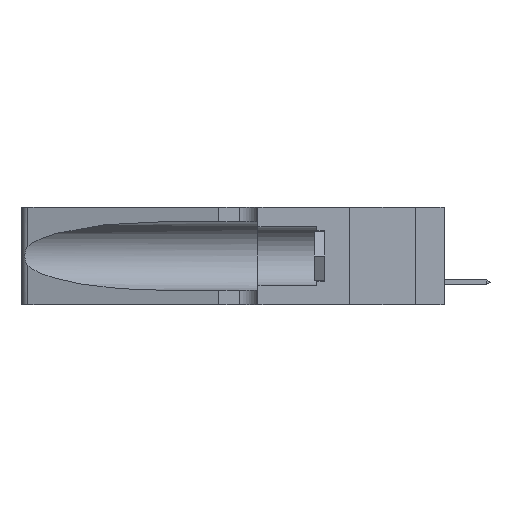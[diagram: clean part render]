
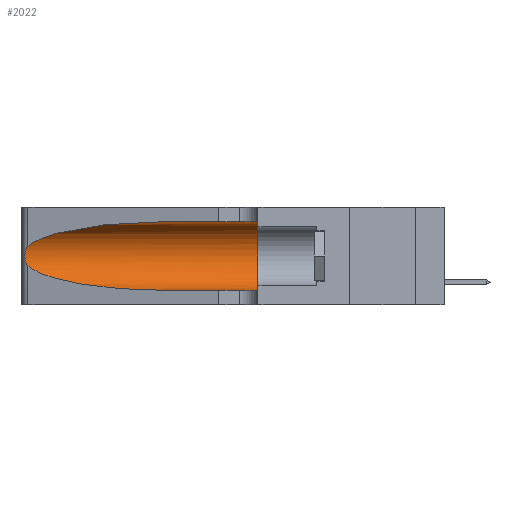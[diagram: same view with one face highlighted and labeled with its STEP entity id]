
A CAD part, left-side view. The second image highlights one B-rep face of the part: STEP entity #2022.
In plain terms, the highlighted cylindrical face has radius 3.308 mm (diameter 6.617 mm), a partial arc.
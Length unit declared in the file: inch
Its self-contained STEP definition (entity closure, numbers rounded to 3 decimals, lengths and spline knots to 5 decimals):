
#895 = CARTESIAN_POINT ( 'NONE',  ( 0.26075, 1.23896, 0.178 ) ) ;
#1084 = CARTESIAN_POINT ( 'NONE',  ( 0.25789, 1.23486, 0.15765 ) ) ;
#1681 = CARTESIAN_POINT ( 'NONE',  ( 0.1305, 1.61858, 0.05475 ) ) ;
#2022 = ADVANCED_FACE ( 'NONE', ( #19001 ), #25500, .F. ) ;
#2192 = CARTESIAN_POINT ( 'NONE',  ( 0.1305, 0.35, 0.31525 ) ) ;
#3175 = CARTESIAN_POINT ( 'NONE',  ( 0.26017, 1.23833, 0.17102 ) ) ;
#3260 = CARTESIAN_POINT ( 'NONE',  ( 0.25487, 1.22718, 0.22369 ) ) ;
#3680 = CARTESIAN_POINT ( 'NONE',  ( 0.18966, 0.96281, 0.05475 ) ) ;
#4371 = EDGE_CURVE ( 'NONE', #13887, #6956, #28282, .T. ) ;
#4872 = DIRECTION ( 'NONE',  ( 0., 1., 0. ) ) ;
#5589 = EDGE_LOOP ( 'NONE', ( #8509, #25087, #11825, #19146, #22375, #6276 ) ) ;
#6276 = ORIENTED_EDGE ( 'NONE', *, *, #19593, .F. ) ;
#6299 = CARTESIAN_POINT ( 'NONE',  ( 0.1305, 0.72297, 0.31525 ) ) ;
#6349 = AXIS2_PLACEMENT_3D ( 'NONE', #23800, #17029, #8109 ) ;
#6956 = VERTEX_POINT ( 'NONE', #27412 ) ;
#7558 = CARTESIAN_POINT ( 'NONE',  ( 0.25555, 1.22993, 0.14849 ) ) ;
#7733 = CARTESIAN_POINT ( 'NONE',  ( 0.1305, 0.72297, 0.31525 ) ) ;
#8109 = DIRECTION ( 'NONE',  ( 0., 0., -1. ) ) ;
#8509 = ORIENTED_EDGE ( 'NONE', *, *, #13877, .T. ) ;
#8916 =( BOUNDED_CURVE ( )  B_SPLINE_CURVE ( 3, ( #16526, #25225, #3680, #21270 ),
 .UNSPECIFIED., .F., .F. ) 
 B_SPLINE_CURVE_WITH_KNOTS ( ( 4, 4 ),
 ( 3.44316, 4.71239 ),
 .UNSPECIFIED. ) 
 CURVE ( )  GEOMETRIC_REPRESENTATION_ITEM ( )  RATIONAL_B_SPLINE_CURVE ( ( 1., 0.87, 0.87, 1. ) ) 
 REPRESENTATION_ITEM ( '' )  );
#9267 = B_SPLINE_CURVE_WITH_KNOTS ( 'NONE', 3,
 ( #3260, #11821, #18405, #27222, #18689, #11726, #27312, #895, #3175, #18597, #1084, #20752, #7558, #9755 ),
 .UNSPECIFIED., .F., .F.,
 ( 4, 2, 2, 2, 2, 2, 4 ),
 ( 0., 0.00027, 0.00053, 0.00107, 0.0016, 0.00187, 0.00214 ),
 .UNSPECIFIED. ) ;
#9755 = CARTESIAN_POINT ( 'NONE',  ( 0.25487, 1.22718, 0.14631 ) ) ;
#10133 = CARTESIAN_POINT ( 'NONE',  ( 0.1305, 0.72297, 0.05475 ) ) ;
#10475 = DIRECTION ( 'NONE',  ( 0., -1., 0. ) ) ;
#10984 = AXIS2_PLACEMENT_3D ( 'NONE', #11786, #4872, #26999 ) ;
#11726 = CARTESIAN_POINT ( 'NONE',  ( 0.26018, 1.23835, 0.19895 ) ) ;
#11786 = CARTESIAN_POINT ( 'NONE',  ( 0.1305, 0.35, 0.185 ) ) ;
#11821 = CARTESIAN_POINT ( 'NONE',  ( 0.25555, 1.22994, 0.2215 ) ) ;
#11825 = ORIENTED_EDGE ( 'NONE', *, *, #28073, .T. ) ;
#12923 = CARTESIAN_POINT ( 'NONE',  ( 0.2373, 1.15595, 0.28018 ) ) ;
#13802 = VERTEX_POINT ( 'NONE', #10133 ) ;
#13877 = EDGE_CURVE ( 'NONE', #22145, #16913, #20389, .T. ) ;
#13887 = VERTEX_POINT ( 'NONE', #2192 ) ;
#14227 = EDGE_CURVE ( 'NONE', #13802, #6956, #16659, .T. ) ;
#14651 = CARTESIAN_POINT ( 'NONE',  ( 0.1305, 1.61858, 0.31525 ) ) ;
#14879 = CARTESIAN_POINT ( 'NONE',  ( 0.25487, 1.22718, 0.14631 ) ) ;
#15415 = VECTOR ( 'NONE', #19107, 39.37008 ) ;
#15669 = CARTESIAN_POINT ( 'NONE',  ( 0.25487, 1.22718, 0.22369 ) ) ;
#15785 = LINE ( 'NONE', #14651, #15415 ) ;
#16526 = CARTESIAN_POINT ( 'NONE',  ( 0.25487, 1.22718, 0.14631 ) ) ;
#16659 = LINE ( 'NONE', #1681, #26252 ) ;
#16913 = VERTEX_POINT ( 'NONE', #15669 ) ;
#17029 = DIRECTION ( 'NONE',  ( 0., -1., 0. ) ) ;
#18405 = CARTESIAN_POINT ( 'NONE',  ( 0.25639, 1.23184, 0.21858 ) ) ;
#18597 = CARTESIAN_POINT ( 'NONE',  ( 0.25856, 1.23593, 0.16098 ) ) ;
#18689 = CARTESIAN_POINT ( 'NONE',  ( 0.25854, 1.2359, 0.20912 ) ) ;
#19001 = FACE_OUTER_BOUND ( 'NONE', #5589, .T. ) ;
#19107 = DIRECTION ( 'NONE',  ( 0., -1., 0. ) ) ;
#19146 = ORIENTED_EDGE ( 'NONE', *, *, #14227, .T. ) ;
#19593 = EDGE_CURVE ( 'NONE', #22145, #13887, #15785, .T. ) ;
#19798 = EDGE_CURVE ( 'NONE', #16913, #27651, #9267, .T. ) ;
#20389 =( BOUNDED_CURVE ( )  B_SPLINE_CURVE ( 3, ( #6299, #23693, #12923, #24080 ),
 .UNSPECIFIED., .F., .T. ) 
 B_SPLINE_CURVE_WITH_KNOTS ( ( 4, 4 ),
 ( 1.5708, 2.84003 ),
 .UNSPECIFIED. ) 
 CURVE ( )  GEOMETRIC_REPRESENTATION_ITEM ( )  RATIONAL_B_SPLINE_CURVE ( ( 1., 0.87, 0.87, 1. ) ) 
 REPRESENTATION_ITEM ( '' )  );
#20752 = CARTESIAN_POINT ( 'NONE',  ( 0.25639, 1.23186, 0.15144 ) ) ;
#21270 = CARTESIAN_POINT ( 'NONE',  ( 0.1305, 0.72297, 0.05475 ) ) ;
#22145 = VERTEX_POINT ( 'NONE', #7733 ) ;
#22375 = ORIENTED_EDGE ( 'NONE', *, *, #4371, .F. ) ;
#23693 = CARTESIAN_POINT ( 'NONE',  ( 0.18966, 0.96281, 0.31525 ) ) ;
#23800 = CARTESIAN_POINT ( 'NONE',  ( 0.1305, 1.61858, 0.185 ) ) ;
#24080 = CARTESIAN_POINT ( 'NONE',  ( 0.25487, 1.22718, 0.22369 ) ) ;
#25087 = ORIENTED_EDGE ( 'NONE', *, *, #19798, .T. ) ;
#25225 = CARTESIAN_POINT ( 'NONE',  ( 0.2373, 1.15595, 0.08982 ) ) ;
#25500 = CYLINDRICAL_SURFACE ( 'NONE', #6349, 0.13025 ) ;
#26252 = VECTOR ( 'NONE', #10475, 39.37008 ) ;
#26999 = DIRECTION ( 'NONE',  ( 0., 0., 1. ) ) ;
#27222 = CARTESIAN_POINT ( 'NONE',  ( 0.25787, 1.23484, 0.2124 ) ) ;
#27312 = CARTESIAN_POINT ( 'NONE',  ( 0.26075, 1.23896, 0.19203 ) ) ;
#27412 = CARTESIAN_POINT ( 'NONE',  ( 0.1305, 0.35, 0.05475 ) ) ;
#27651 = VERTEX_POINT ( 'NONE', #14879 ) ;
#28073 = EDGE_CURVE ( 'NONE', #27651, #13802, #8916, .T. ) ;
#28282 = CIRCLE ( 'NONE', #10984, 0.13025 ) ;
